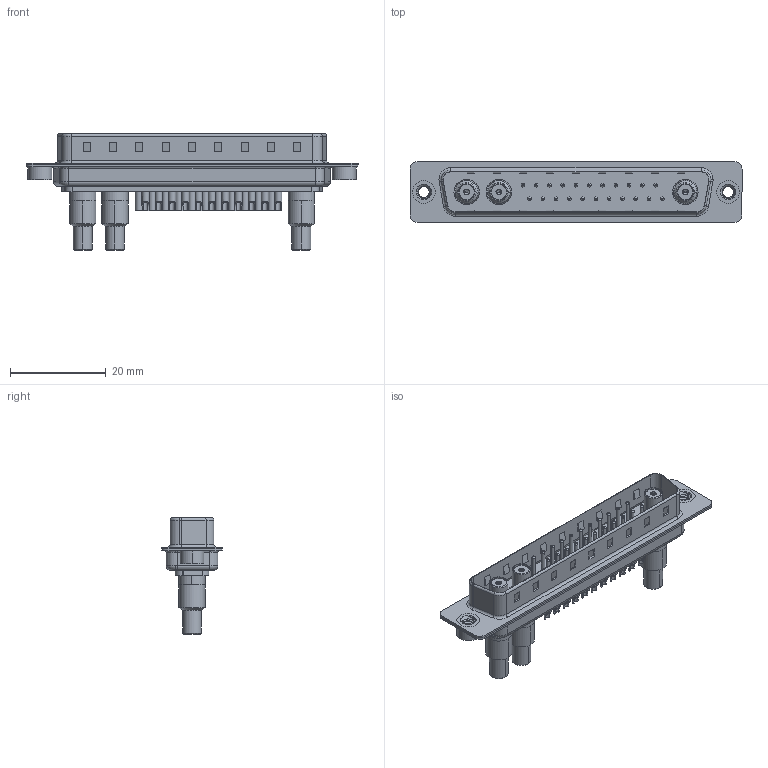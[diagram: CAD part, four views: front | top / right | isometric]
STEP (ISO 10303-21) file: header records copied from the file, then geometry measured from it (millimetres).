
FILE_DESCRIPTION (( 'STEP AP203' ), '1' );
FILE_NAME ('627-25W3622-5N2.STEP', '2019-05-29T21:04:03', ( '' ), ( '' ), 'SwSTEP 2.0', 'SolidWorks 2016', '' );
FILE_SCHEMA (( 'CONFIG_CONTROL_DESIGN' ));
Length unit declared in the file: millimetre
Products named in the file (14): Locking Collar; Socket_Solder Cup; 627Combo Housing_25W3; Solder Cover; 627Combo Shell Rear_37 Contacts; Co-Ax Jack Assy_SC; 627Combo Shell Front_37 Contacts; 627Combo Contact Row 1_22; 627Combo Threaded Rivet_2; 627Combo Contact Row 2_22; Co-Ax Jack_Solder Cup Tail; 627-25W3622-5N2; Insulator Socket; Insulator Socket 2
Assembly tree (36 placements, depth 3):
  627-25W3622-5N2
    627Combo Housing_25W3
    627Combo Shell Rear_37 Contacts
    627Combo Shell Front_37 Contacts
    627Combo Threaded Rivet_2  x2
    Co-Ax Jack Assy_SC  x3
      Co-Ax Jack_Solder Cup Tail
      Insulator Socket
      Insulator Socket 2
      Locking Collar
      Socket_Solder Cup
      Solder Cover
    627Combo Contact Row 1_22  x11
    627Combo Contact Row 2_22  x11
Bounding box: 69.3 x 12.6 x 24.3 mm (x, y, z)
Volume: 4182.9 mm3; surface area: 11864.6 mm2
Topology: 45 solids, 45 shells, 1616 faces, 3772 edges, 2316 vertices
Faces by surface type: cylinder 685, plane 521, torus 282, cone 116, bspline 12
Entity records: 25948 total; most frequent: CARTESIAN_POINT 5482, DIRECTION 4097, ORIENTED_EDGE 3614, EDGE_CURVE 1807, AXIS2_PLACEMENT_3D 1583, VERTEX_POINT 1148, EDGE_LOOP 933, VECTOR 931
